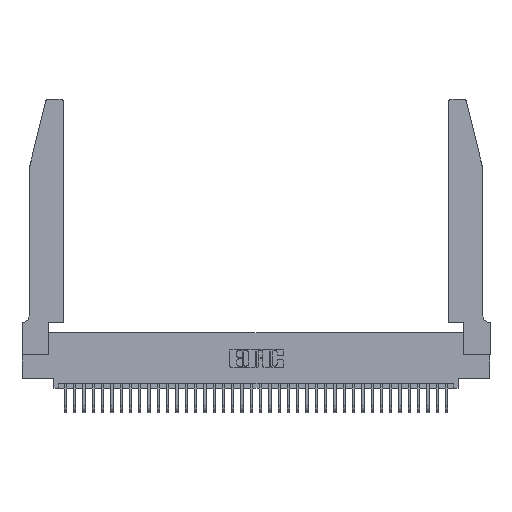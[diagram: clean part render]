
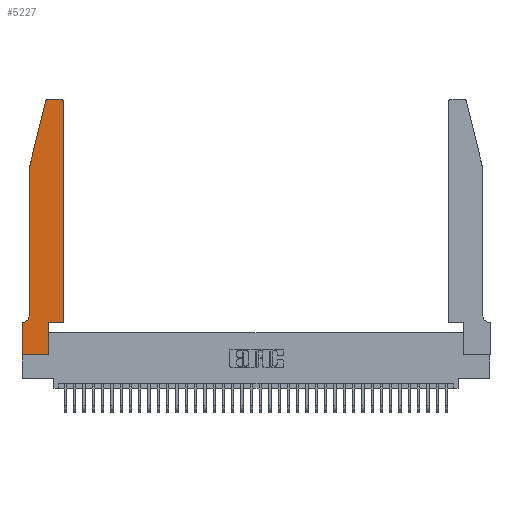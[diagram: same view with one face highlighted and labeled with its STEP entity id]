
A CAD part, top view. The second image highlights one B-rep face of the part: STEP entity #5227.
In plain terms, the highlighted planar face has unit normal (0, 0, 1).
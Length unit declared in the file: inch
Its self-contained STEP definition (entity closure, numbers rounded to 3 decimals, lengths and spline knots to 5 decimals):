
#18 = ORIENTED_EDGE ( 'NONE', *, *, #38404, .T. ) ;
#536 = VECTOR ( 'NONE', #29351, 39.37008 ) ;
#624 = VECTOR ( 'NONE', #22629, 39.37008 ) ;
#635 = LINE ( 'NONE', #28567, #24194 ) ;
#1780 = CARTESIAN_POINT ( 'NONE',  ( 0.0755, 2., 0.37 ) ) ;
#2000 = CARTESIAN_POINT ( 'NONE',  ( 0.0055, 0.35, 0.37 ) ) ;
#2121 = CARTESIAN_POINT ( 'NONE',  ( 0.4505, 2.72, 0.37 ) ) ;
#2170 = EDGE_CURVE ( 'NONE', #21005, #7629, #31645, .T. ) ;
#2513 = EDGE_LOOP ( 'NONE', ( #34433, #37693, #18302, #14100, #18651, #10727, #18, #34511, #37326, #24095, #34053, #12675 ) ) ;
#3083 = CARTESIAN_POINT ( 'NONE',  ( 0.0755, 2., 0.37 ) ) ;
#3674 = EDGE_CURVE ( 'NONE', #19592, #9723, #10844, .T. ) ;
#4064 = CIRCLE ( 'NONE', #28060, 0.07 ) ;
#4331 = EDGE_CURVE ( 'NONE', #11709, #39212, #9919, .T. ) ;
#5227 = ADVANCED_FACE ( 'NONE', ( #35956 ), #12655, .T. ) ;
#5652 = CARTESIAN_POINT ( 'NONE',  ( 0.0755, 2., 0.37 ) ) ;
#6247 = LINE ( 'NONE', #38762, #22508 ) ;
#6486 = CARTESIAN_POINT ( 'NONE',  ( 0., 0.35, 0.37 ) ) ;
#7063 = VECTOR ( 'NONE', #29028, 39.37008 ) ;
#7182 = LINE ( 'NONE', #3083, #38499 ) ;
#7629 = VERTEX_POINT ( 'NONE', #21057 ) ;
#8035 = LINE ( 'NONE', #26007, #7063 ) ;
#8110 = CARTESIAN_POINT ( 'NONE',  ( 0.0755, 0.42, 0.37 ) ) ;
#8313 = VERTEX_POINT ( 'NONE', #27790 ) ;
#8502 = EDGE_CURVE ( 'NONE', #39212, #18426, #7182, .T. ) ;
#8859 = LINE ( 'NONE', #1780, #536 ) ;
#9288 = DIRECTION ( 'NONE',  ( 0., 0., 1. ) ) ;
#9384 = DIRECTION ( 'NONE',  ( -0.239, -0.971, 0. ) ) ;
#9507 = EDGE_CURVE ( 'NONE', #21047, #26154, #29924, .T. ) ;
#9723 = VERTEX_POINT ( 'NONE', #27373 ) ;
#9919 = CIRCLE ( 'NONE', #31772, 0.03 ) ;
#10273 = DIRECTION ( 'NONE',  ( 0., 0., -1. ) ) ;
#10727 = ORIENTED_EDGE ( 'NONE', *, *, #3674, .T. ) ;
#10844 = LINE ( 'NONE', #16473, #624 ) ;
#10949 = VERTEX_POINT ( 'NONE', #17703 ) ;
#11483 = DIRECTION ( 'NONE',  ( 1., 0., 0. ) ) ;
#11709 = VERTEX_POINT ( 'NONE', #15537 ) ;
#12069 = EDGE_CURVE ( 'NONE', #18426, #30046, #8859, .T. ) ;
#12655 = PLANE ( 'NONE',  #19310 ) ;
#12675 = ORIENTED_EDGE ( 'NONE', *, *, #2170, .T. ) ;
#14100 = ORIENTED_EDGE ( 'NONE', *, *, #12069, .T. ) ;
#14371 = DIRECTION ( 'NONE',  ( 1., 0., 0. ) ) ;
#14483 = CARTESIAN_POINT ( 'NONE',  ( 0.2605, 2.75, 0.37 ) ) ;
#14791 = CARTESIAN_POINT ( 'NONE',  ( 0.2865, 0.35, 0.37 ) ) ;
#14810 = DIRECTION ( 'NONE',  ( 0., 1., 0. ) ) ;
#15537 = CARTESIAN_POINT ( 'NONE',  ( 0.284, 2.75, 0.37 ) ) ;
#15684 = DIRECTION ( 'NONE',  ( 1., 0., 0. ) ) ;
#16473 = CARTESIAN_POINT ( 'NONE',  ( 0.0755, 0.35, 0.37 ) ) ;
#17349 = DIRECTION ( 'NONE',  ( 0., 0., 1. ) ) ;
#17505 = DIRECTION ( 'NONE',  ( -1., 0., 0. ) ) ;
#17532 = CARTESIAN_POINT ( 'NONE',  ( 0.25487, 2.72718, 0.37 ) ) ;
#17703 = CARTESIAN_POINT ( 'NONE',  ( 0., 0., 0.37 ) ) ;
#18302 = ORIENTED_EDGE ( 'NONE', *, *, #8502, .T. ) ;
#18426 = VERTEX_POINT ( 'NONE', #5652 ) ;
#18435 = LINE ( 'NONE', #14483, #35544 ) ;
#18651 = ORIENTED_EDGE ( 'NONE', *, *, #38927, .T. ) ;
#19310 = AXIS2_PLACEMENT_3D ( 'NONE', #6486, #33902, #15684 ) ;
#19395 = DIRECTION ( 'NONE',  ( 0., 1., 0. ) ) ;
#19592 = VERTEX_POINT ( 'NONE', #2000 ) ;
#19630 = EDGE_CURVE ( 'NONE', #10949, #8313, #6247, .T. ) ;
#21005 = VERTEX_POINT ( 'NONE', #2121 ) ;
#21047 = VERTEX_POINT ( 'NONE', #14791 ) ;
#21057 = CARTESIAN_POINT ( 'NONE',  ( 0.4205, 2.75, 0.37 ) ) ;
#22086 = AXIS2_PLACEMENT_3D ( 'NONE', #27475, #9288, #30528 ) ;
#22508 = VECTOR ( 'NONE', #11483, 39.37008 ) ;
#22629 = DIRECTION ( 'NONE',  ( -1., 0., 0. ) ) ;
#23448 = EDGE_CURVE ( 'NONE', #8313, #21047, #25975, .T. ) ;
#24095 = ORIENTED_EDGE ( 'NONE', *, *, #9507, .T. ) ;
#24194 = VECTOR ( 'NONE', #19395, 39.37008 ) ;
#25031 = VECTOR ( 'NONE', #14810, 39.37008 ) ;
#25975 = LINE ( 'NONE', #38901, #25031 ) ;
#26007 = CARTESIAN_POINT ( 'NONE',  ( 0., 0., 0.37 ) ) ;
#26154 = VERTEX_POINT ( 'NONE', #33754 ) ;
#27373 = CARTESIAN_POINT ( 'NONE',  ( 0., 0.35, 0.37 ) ) ;
#27475 = CARTESIAN_POINT ( 'NONE',  ( 0.4205, 2.72, 0.37 ) ) ;
#27790 = CARTESIAN_POINT ( 'NONE',  ( 0.2865, 0., 0.37 ) ) ;
#28060 = AXIS2_PLACEMENT_3D ( 'NONE', #28460, #10273, #31518 ) ;
#28460 = CARTESIAN_POINT ( 'NONE',  ( 0.0055, 0.42, 0.37 ) ) ;
#28551 = EDGE_CURVE ( 'NONE', #26154, #21005, #635, .T. ) ;
#28567 = CARTESIAN_POINT ( 'NONE',  ( 0.4505, 0.35, 0.37 ) ) ;
#28733 = EDGE_CURVE ( 'NONE', #7629, #11709, #18435, .T. ) ;
#28969 = VECTOR ( 'NONE', #14371, 39.37008 ) ;
#29028 = DIRECTION ( 'NONE',  ( 0., -1., 0. ) ) ;
#29351 = DIRECTION ( 'NONE',  ( 0., -1., 0. ) ) ;
#29924 = LINE ( 'NONE', #38460, #28969 ) ;
#30046 = VERTEX_POINT ( 'NONE', #8110 ) ;
#30528 = DIRECTION ( 'NONE',  ( 1., 0., 0. ) ) ;
#31518 = DIRECTION ( 'NONE',  ( -1., 0., 0. ) ) ;
#31645 = CIRCLE ( 'NONE', #22086, 0.03 ) ;
#31772 = AXIS2_PLACEMENT_3D ( 'NONE', #35543, #17349, #38533 ) ;
#33754 = CARTESIAN_POINT ( 'NONE',  ( 0.4505, 0.35, 0.37 ) ) ;
#33902 = DIRECTION ( 'NONE',  ( 0., 0., 1. ) ) ;
#34053 = ORIENTED_EDGE ( 'NONE', *, *, #28551, .T. ) ;
#34433 = ORIENTED_EDGE ( 'NONE', *, *, #28733, .T. ) ;
#34511 = ORIENTED_EDGE ( 'NONE', *, *, #19630, .T. ) ;
#35543 = CARTESIAN_POINT ( 'NONE',  ( 0.284, 2.72, 0.37 ) ) ;
#35544 = VECTOR ( 'NONE', #17505, 39.37008 ) ;
#35956 = FACE_OUTER_BOUND ( 'NONE', #2513, .T. ) ;
#37326 = ORIENTED_EDGE ( 'NONE', *, *, #23448, .T. ) ;
#37693 = ORIENTED_EDGE ( 'NONE', *, *, #4331, .T. ) ;
#38404 = EDGE_CURVE ( 'NONE', #9723, #10949, #8035, .T. ) ;
#38460 = CARTESIAN_POINT ( 'NONE',  ( 0.4505, 0.35, 0.37 ) ) ;
#38499 = VECTOR ( 'NONE', #9384, 39.37008 ) ;
#38533 = DIRECTION ( 'NONE',  ( 1., 0., 0. ) ) ;
#38762 = CARTESIAN_POINT ( 'NONE',  ( 0., 0., 0.37 ) ) ;
#38901 = CARTESIAN_POINT ( 'NONE',  ( 0.2865, 0.35, 0.37 ) ) ;
#38927 = EDGE_CURVE ( 'NONE', #30046, #19592, #4064, .T. ) ;
#39212 = VERTEX_POINT ( 'NONE', #17532 ) ;
